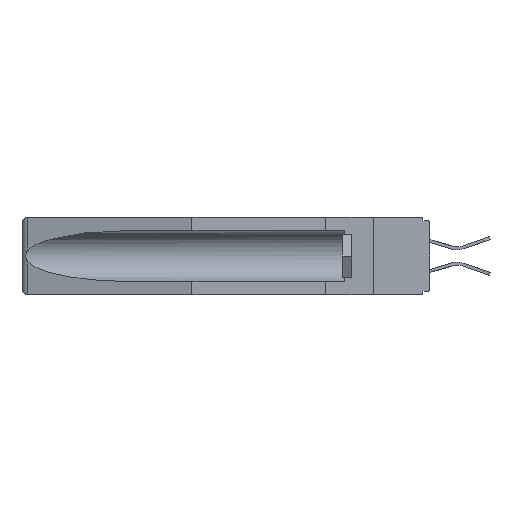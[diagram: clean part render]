
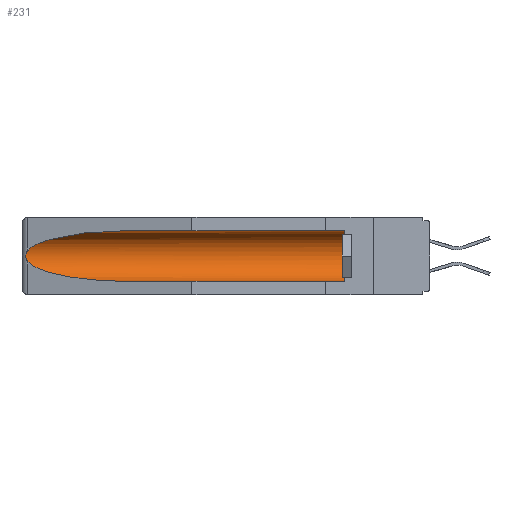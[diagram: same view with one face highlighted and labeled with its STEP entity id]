
A CAD part, left-side view. The second image highlights one B-rep face of the part: STEP entity #231.
In plain terms, the highlighted cylindrical face has radius 2.857 mm (diameter 5.715 mm), a partial arc.
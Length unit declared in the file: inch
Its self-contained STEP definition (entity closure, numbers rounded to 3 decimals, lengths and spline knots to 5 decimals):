
#231 = ADVANCED_FACE ( 'NONE', ( #11790 ), #15046, .F. ) ;
#335 = EDGE_CURVE ( 'NONE', #29978, #22989, #26679, .T. ) ;
#798 = CARTESIAN_POINT ( 'NONE',  ( 0.155, -0.30754, -0.059 ) ) ;
#1890 = VERTEX_POINT ( 'NONE', #2964 ) ;
#2027 = CARTESIAN_POINT ( 'NONE',  ( 0.155, 1.07973, -0.059 ) ) ;
#2229 = CARTESIAN_POINT ( 'NONE',  ( 0.25451, 1.48313, -0.09465 ) ) ;
#2650 = CARTESIAN_POINT ( 'NONE',  ( 0.26537, 1.52718, -0.19328 ) ) ;
#2964 = CARTESIAN_POINT ( 'NONE',  ( 0.155, 0.126, -0.059 ) ) ;
#3031 = LINE ( 'NONE', #3793, #21673 ) ;
#3557 = DIRECTION ( 'NONE',  ( 0., -1., 0. ) ) ;
#3793 = CARTESIAN_POINT ( 'NONE',  ( 0.155, -0.30754, -0.284 ) ) ;
#3952 = VERTEX_POINT ( 'NONE', #25492 ) ;
#4399 = EDGE_CURVE ( 'NONE', #22989, #24357, #13033, .T. ) ;
#5797 = LINE ( 'NONE', #798, #6536 ) ;
#5907 = CARTESIAN_POINT ( 'NONE',  ( 0.26537, 1.52718, -0.19328 ) ) ;
#5913 = CARTESIAN_POINT ( 'NONE',  ( 0.155, 0.126, -0.1715 ) ) ;
#6090 = EDGE_CURVE ( 'NONE', #3952, #29978, #15810, .T. ) ;
#6536 = VECTOR ( 'NONE', #12449, 39.37008 ) ;
#6552 = ORIENTED_EDGE ( 'NONE', *, *, #6090, .T. ) ;
#6719 = CARTESIAN_POINT ( 'NONE',  ( 0.26537, 1.52718, -0.14972 ) ) ;
#7928 = CARTESIAN_POINT ( 'NONE',  ( 0.26597, 1.5296, -0.19026 ) ) ;
#8406 = AXIS2_PLACEMENT_3D ( 'NONE', #5913, #3557, #10609 ) ;
#9288 = ORIENTED_EDGE ( 'NONE', *, *, #24671, .F. ) ;
#9698 = CARTESIAN_POINT ( 'NONE',  ( 0.155, 1.07973, -0.284 ) ) ;
#10165 = EDGE_LOOP ( 'NONE', ( #6552, #24485, #11837, #9288, #28575, #26198 ) ) ;
#10182 = CARTESIAN_POINT ( 'NONE',  ( 0.2675, 1.53308, -0.17534 ) ) ;
#10190 = CIRCLE ( 'NONE', #8406, 0.1125 ) ;
#10609 = DIRECTION ( 'NONE',  ( 0., 0., 1. ) ) ;
#10698 = AXIS2_PLACEMENT_3D ( 'NONE', #17993, #29623, #13282 ) ;
#11059 = CARTESIAN_POINT ( 'NONE',  ( 0.26537, 1.52718, -0.14972 ) ) ;
#11790 = FACE_OUTER_BOUND ( 'NONE', #10165, .T. ) ;
#11837 = ORIENTED_EDGE ( 'NONE', *, *, #4399, .T. ) ;
#12449 = DIRECTION ( 'NONE',  ( 0., 1., 0. ) ) ;
#13033 =( BOUNDED_CURVE ( )  B_SPLINE_CURVE ( 3, ( #20805, #20590, #18524, #20485 ),
 .UNSPECIFIED., .F., .F. ) 
 B_SPLINE_CURVE_WITH_KNOTS ( ( 4, 4 ),
 ( 0.1948, 1.5708 ),
 .UNSPECIFIED. ) 
 CURVE ( )  GEOMETRIC_REPRESENTATION_ITEM ( )  RATIONAL_B_SPLINE_CURVE ( ( 1., 0.848, 0.848, 1. ) ) 
 REPRESENTATION_ITEM ( '' )  );
#13282 = DIRECTION ( 'NONE',  ( 0., 0., 1. ) ) ;
#13688 = EDGE_CURVE ( 'NONE', #20121, #1890, #10190, .T. ) ;
#15046 = CYLINDRICAL_SURFACE ( 'NONE', #10698, 0.1125 ) ;
#15406 = CARTESIAN_POINT ( 'NONE',  ( 0.2675, 1.53308, -0.16763 ) ) ;
#15810 =( BOUNDED_CURVE ( )  B_SPLINE_CURVE ( 3, ( #2027, #30233, #2229, #6719 ),
 .UNSPECIFIED., .F., .F. ) 
 B_SPLINE_CURVE_WITH_KNOTS ( ( 4, 4 ),
 ( 4.71239, 6.08839 ),
 .UNSPECIFIED. ) 
 CURVE ( )  GEOMETRIC_REPRESENTATION_ITEM ( )  RATIONAL_B_SPLINE_CURVE ( ( 1., 0.848, 0.848, 1. ) ) 
 REPRESENTATION_ITEM ( '' )  );
#16432 = CARTESIAN_POINT ( 'NONE',  ( 0.26537, 1.52718, -0.14972 ) ) ;
#17993 = CARTESIAN_POINT ( 'NONE',  ( 0.155, -0.30754, -0.1715 ) ) ;
#18524 = CARTESIAN_POINT ( 'NONE',  ( 0.21114, 1.30732, -0.284 ) ) ;
#20121 = VERTEX_POINT ( 'NONE', #26956 ) ;
#20485 = CARTESIAN_POINT ( 'NONE',  ( 0.155, 1.07973, -0.284 ) ) ;
#20590 = CARTESIAN_POINT ( 'NONE',  ( 0.25451, 1.48313, -0.24835 ) ) ;
#20805 = CARTESIAN_POINT ( 'NONE',  ( 0.26537, 1.52718, -0.19328 ) ) ;
#21490 = CARTESIAN_POINT ( 'NONE',  ( 0.26654, 1.53092, -0.15636 ) ) ;
#21673 = VECTOR ( 'NONE', #24852, 39.37008 ) ;
#22989 = VERTEX_POINT ( 'NONE', #2650 ) ;
#24314 = CARTESIAN_POINT ( 'NONE',  ( 0.2673, 1.5327, -0.16383 ) ) ;
#24357 = VERTEX_POINT ( 'NONE', #9698 ) ;
#24485 = ORIENTED_EDGE ( 'NONE', *, *, #335, .T. ) ;
#24671 = EDGE_CURVE ( 'NONE', #20121, #24357, #3031, .T. ) ;
#24852 = DIRECTION ( 'NONE',  ( 0., 1., 0. ) ) ;
#25492 = CARTESIAN_POINT ( 'NONE',  ( 0.155, 1.07973, -0.059 ) ) ;
#26198 = ORIENTED_EDGE ( 'NONE', *, *, #29163, .T. ) ;
#26573 = CARTESIAN_POINT ( 'NONE',  ( 0.26655, 1.53094, -0.18657 ) ) ;
#26679 = B_SPLINE_CURVE_WITH_KNOTS ( 'NONE', 3,
 ( #11059, #27677, #21490, #24314, #15406, #10182, #29140, #26573, #7928, #5907 ),
 .UNSPECIFIED., .F., .F.,
 ( 4, 2, 2, 2, 4 ),
 ( 0., 0.00029, 0.00058, 0.00087, 0.00117 ),
 .UNSPECIFIED. ) ;
#26956 = CARTESIAN_POINT ( 'NONE',  ( 0.155, 0.126, -0.284 ) ) ;
#27677 = CARTESIAN_POINT ( 'NONE',  ( 0.26597, 1.52961, -0.15275 ) ) ;
#28575 = ORIENTED_EDGE ( 'NONE', *, *, #13688, .T. ) ;
#29140 = CARTESIAN_POINT ( 'NONE',  ( 0.2673, 1.53269, -0.17917 ) ) ;
#29163 = EDGE_CURVE ( 'NONE', #1890, #3952, #5797, .T. ) ;
#29623 = DIRECTION ( 'NONE',  ( 0., 1., 0. ) ) ;
#29978 = VERTEX_POINT ( 'NONE', #16432 ) ;
#30233 = CARTESIAN_POINT ( 'NONE',  ( 0.21114, 1.30732, -0.059 ) ) ;
